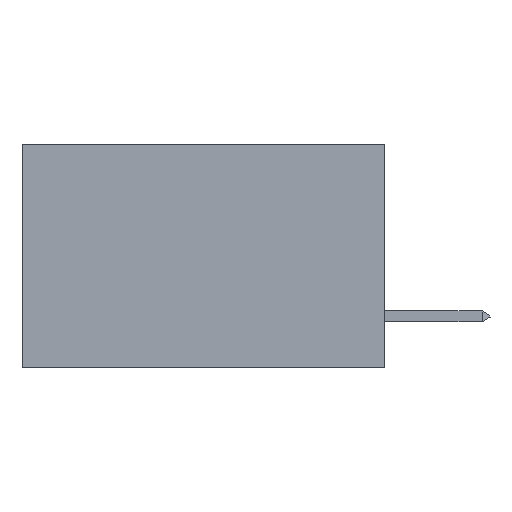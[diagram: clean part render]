
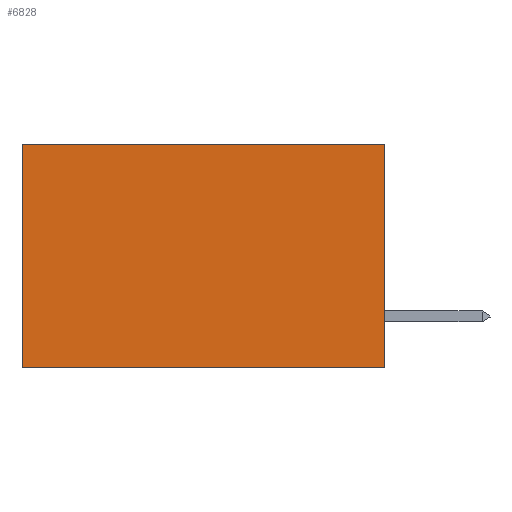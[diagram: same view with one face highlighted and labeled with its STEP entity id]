
A CAD part, left-side view. The second image highlights one B-rep face of the part: STEP entity #6828.
In plain terms, the highlighted planar face has unit normal (-1, 0, 0).
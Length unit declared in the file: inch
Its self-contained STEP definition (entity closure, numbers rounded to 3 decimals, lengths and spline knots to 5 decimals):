
#800 = VERTEX_POINT ( 'NONE', #34663 ) ;
#2488 = ORIENTED_EDGE ( 'NONE', *, *, #36309, .T. ) ;
#2968 = LINE ( 'NONE', #4182, #17459 ) ;
#3602 = VERTEX_POINT ( 'NONE', #27856 ) ;
#4182 = CARTESIAN_POINT ( 'NONE',  ( 0.2875, 0., 0. ) ) ;
#6665 = ORIENTED_EDGE ( 'NONE', *, *, #25692, .F. ) ;
#6828 = ADVANCED_FACE ( 'NONE', ( #17393 ), #25288, .F. ) ;
#8408 = ORIENTED_EDGE ( 'NONE', *, *, #26377, .F. ) ;
#8726 = DIRECTION ( 'NONE',  ( 1., 0., 0. ) ) ;
#9427 = CARTESIAN_POINT ( 'NONE',  ( 0.2875, 0., -0.37 ) ) ;
#9568 = VECTOR ( 'NONE', #33574, 39.37008 ) ;
#9688 = DIRECTION ( 'NONE',  ( 0., 1., 0. ) ) ;
#9734 = CARTESIAN_POINT ( 'NONE',  ( 0.2875, 0., 0. ) ) ;
#10171 = EDGE_LOOP ( 'NONE', ( #2488, #6665, #8408, #25777 ) ) ;
#12723 = VECTOR ( 'NONE', #20983, 39.37008 ) ;
#12862 = CARTESIAN_POINT ( 'NONE',  ( 0.2875, 0., 0. ) ) ;
#13395 = EDGE_CURVE ( 'NONE', #24480, #3602, #2968, .T. ) ;
#15478 = DIRECTION ( 'NONE',  ( 0., 1., 0. ) ) ;
#15798 = LINE ( 'NONE', #9734, #12723 ) ;
#17393 = FACE_OUTER_BOUND ( 'NONE', #10171, .T. ) ;
#17459 = VECTOR ( 'NONE', #15478, 39.37008 ) ;
#20693 = AXIS2_PLACEMENT_3D ( 'NONE', #25521, #8726, #22542 ) ;
#20983 = DIRECTION ( 'NONE',  ( 0., 0., -1. ) ) ;
#22542 = DIRECTION ( 'NONE',  ( 0., 0., -1. ) ) ;
#24480 = VERTEX_POINT ( 'NONE', #12862 ) ;
#24889 = LINE ( 'NONE', #28163, #9568 ) ;
#25032 = LINE ( 'NONE', #9427, #29874 ) ;
#25288 = PLANE ( 'NONE',  #20693 ) ;
#25521 = CARTESIAN_POINT ( 'NONE',  ( 0.2875, 0., 0. ) ) ;
#25692 = EDGE_CURVE ( 'NONE', #29400, #800, #25032, .T. ) ;
#25777 = ORIENTED_EDGE ( 'NONE', *, *, #13395, .T. ) ;
#26377 = EDGE_CURVE ( 'NONE', #24480, #29400, #15798, .T. ) ;
#27856 = CARTESIAN_POINT ( 'NONE',  ( 0.2875, 0.6, 0. ) ) ;
#28163 = CARTESIAN_POINT ( 'NONE',  ( 0.2875, 0.6, 0. ) ) ;
#29400 = VERTEX_POINT ( 'NONE', #31720 ) ;
#29874 = VECTOR ( 'NONE', #9688, 39.37008 ) ;
#31720 = CARTESIAN_POINT ( 'NONE',  ( 0.2875, 0., -0.37 ) ) ;
#33574 = DIRECTION ( 'NONE',  ( 0., 0., -1. ) ) ;
#34663 = CARTESIAN_POINT ( 'NONE',  ( 0.2875, 0.6, -0.37 ) ) ;
#36309 = EDGE_CURVE ( 'NONE', #3602, #800, #24889, .T. ) ;
